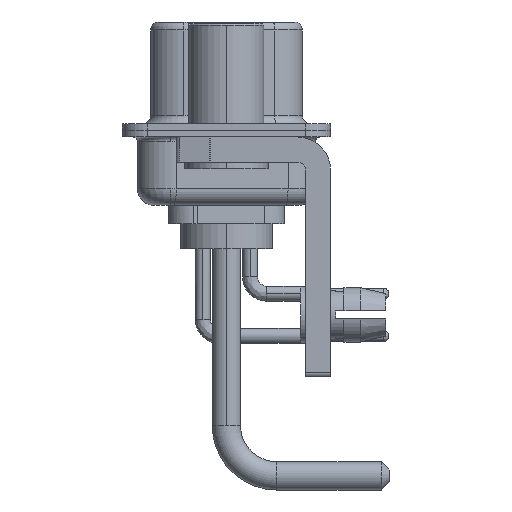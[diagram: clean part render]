
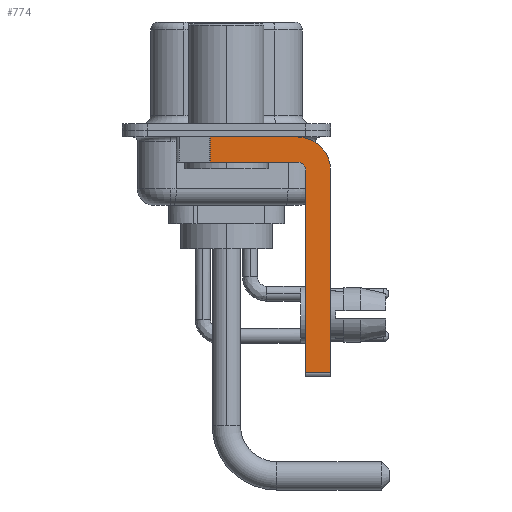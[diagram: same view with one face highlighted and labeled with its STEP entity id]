
A CAD part, left-side view. The second image highlights one B-rep face of the part: STEP entity #774.
In plain terms, the highlighted planar face has unit normal (-1, 0, 0).
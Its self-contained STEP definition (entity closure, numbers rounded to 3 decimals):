
#564 = DIRECTION ( 'NONE',  ( 0., 0., 1. ) ) ;
#774 = ADVANCED_FACE ( 'NONE', ( #10113 ), #27940, .F. ) ;
#1044 = LINE ( 'NONE', #5368, #12003 ) ;
#1234 = ORIENTED_EDGE ( 'NONE', *, *, #3634, .F. ) ;
#1463 = CARTESIAN_POINT ( 'NONE',  ( -2.9, -4.25, -2.4 ) ) ;
#1567 = VERTEX_POINT ( 'NONE', #2811 ) ;
#2404 = AXIS2_PLACEMENT_3D ( 'NONE', #1463, #26087, #26253 ) ;
#2811 = CARTESIAN_POINT ( 'NONE',  ( -2.9, -4.25, -0.4 ) ) ;
#2847 = DIRECTION ( 'NONE',  ( 0., 0., -1. ) ) ;
#3634 = EDGE_CURVE ( 'NONE', #18021, #13394, #13220, .T. ) ;
#4487 = CARTESIAN_POINT ( 'NONE',  ( -2.9, -4.25, -2.4 ) ) ;
#4688 = CARTESIAN_POINT ( 'NONE',  ( -2.9, -4.25, -2.4 ) ) ;
#5109 = CARTESIAN_POINT ( 'NONE',  ( -2.9, -4.25, -1.9 ) ) ;
#5368 = CARTESIAN_POINT ( 'NONE',  ( -2.9, -4.75, -14.8 ) ) ;
#6157 = CARTESIAN_POINT ( 'NONE',  ( -2.9, -4.25, -1.9 ) ) ;
#6579 = ORIENTED_EDGE ( 'NONE', *, *, #14877, .F. ) ;
#6624 = DIRECTION ( 'NONE',  ( 0., -1., 0. ) ) ;
#7213 = ORIENTED_EDGE ( 'NONE', *, *, #32289, .F. ) ;
#7903 = VERTEX_POINT ( 'NONE', #11175 ) ;
#8265 = DIRECTION ( 'NONE',  ( 0., 0., -1. ) ) ;
#8285 = AXIS2_PLACEMENT_3D ( 'NONE', #4688, #25480, #2847 ) ;
#8656 = ORIENTED_EDGE ( 'NONE', *, *, #25302, .T. ) ;
#8937 = LINE ( 'NONE', #11593, #17824 ) ;
#9923 = EDGE_CURVE ( 'NONE', #20042, #30696, #11492, .T. ) ;
#10113 = FACE_OUTER_BOUND ( 'NONE', #10461, .T. ) ;
#10461 = EDGE_LOOP ( 'NONE', ( #28764, #23214, #7213, #27633, #17973, #8656, #1234, #6579 ) ) ;
#10996 = VECTOR ( 'NONE', #23599, 1000. ) ;
#11175 = CARTESIAN_POINT ( 'NONE',  ( -2.9, -4.75, -14.55 ) ) ;
#11492 = LINE ( 'NONE', #26179, #30170 ) ;
#11593 = CARTESIAN_POINT ( 'NONE',  ( -2.9, 3., -0.4 ) ) ;
#12003 = VECTOR ( 'NONE', #564, 1000. ) ;
#13220 = LINE ( 'NONE', #27942, #19456 ) ;
#13394 = VERTEX_POINT ( 'NONE', #15783 ) ;
#14877 = EDGE_CURVE ( 'NONE', #1567, #18021, #15669, .T. ) ;
#15023 = LINE ( 'NONE', #5109, #27027 ) ;
#15160 = EDGE_CURVE ( 'NONE', #29015, #21224, #16746, .T. ) ;
#15669 = CIRCLE ( 'NONE', #8285, 2. ) ;
#15738 = CARTESIAN_POINT ( 'NONE',  ( -2.9, 0.978, -0.4 ) ) ;
#15783 = CARTESIAN_POINT ( 'NONE',  ( -2.9, -6.25, -14.55 ) ) ;
#16746 = CIRCLE ( 'NONE', #17805, 0.5 ) ;
#16793 = EDGE_CURVE ( 'NONE', #7903, #29015, #1044, .T. ) ;
#17805 = AXIS2_PLACEMENT_3D ( 'NONE', #4487, #26945, #26785 ) ;
#17824 = VECTOR ( 'NONE', #6624, 1000. ) ;
#17973 = ORIENTED_EDGE ( 'NONE', *, *, #16793, .F. ) ;
#18021 = VERTEX_POINT ( 'NONE', #31630 ) ;
#18334 = LINE ( 'NONE', #28401, #10996 ) ;
#19456 = VECTOR ( 'NONE', #8265, 1000. ) ;
#20042 = VERTEX_POINT ( 'NONE', #15738 ) ;
#21224 = VERTEX_POINT ( 'NONE', #6157 ) ;
#23214 = ORIENTED_EDGE ( 'NONE', *, *, #9923, .T. ) ;
#23441 = CARTESIAN_POINT ( 'NONE',  ( -2.9, 0.978, -1.9 ) ) ;
#23599 = DIRECTION ( 'NONE',  ( 0., -1., 0. ) ) ;
#23841 = CARTESIAN_POINT ( 'NONE',  ( -2.9, -4.75, -2.4 ) ) ;
#24779 = EDGE_CURVE ( 'NONE', #20042, #1567, #8937, .T. ) ;
#25302 = EDGE_CURVE ( 'NONE', #7903, #13394, #18334, .T. ) ;
#25480 = DIRECTION ( 'NONE',  ( 1., 0., 0. ) ) ;
#26087 = DIRECTION ( 'NONE',  ( 1., 0., 0. ) ) ;
#26179 = CARTESIAN_POINT ( 'NONE',  ( -2.9, 0.978, -1.9 ) ) ;
#26253 = DIRECTION ( 'NONE',  ( 0., 0., -1. ) ) ;
#26785 = DIRECTION ( 'NONE',  ( 0., 0., 1. ) ) ;
#26945 = DIRECTION ( 'NONE',  ( -1., 0., 0. ) ) ;
#27027 = VECTOR ( 'NONE', #27573, 1000. ) ;
#27573 = DIRECTION ( 'NONE',  ( 0., 1., 0. ) ) ;
#27633 = ORIENTED_EDGE ( 'NONE', *, *, #15160, .F. ) ;
#27940 = PLANE ( 'NONE',  #2404 ) ;
#27942 = CARTESIAN_POINT ( 'NONE',  ( -2.9, -6.25, -2.4 ) ) ;
#28401 = CARTESIAN_POINT ( 'NONE',  ( -2.9, -4.25, -14.55 ) ) ;
#28764 = ORIENTED_EDGE ( 'NONE', *, *, #24779, .F. ) ;
#29015 = VERTEX_POINT ( 'NONE', #23841 ) ;
#30170 = VECTOR ( 'NONE', #31140, 1000. ) ;
#30696 = VERTEX_POINT ( 'NONE', #23441 ) ;
#31140 = DIRECTION ( 'NONE',  ( 0., 0., -1. ) ) ;
#31630 = CARTESIAN_POINT ( 'NONE',  ( -2.9, -6.25, -2.4 ) ) ;
#32289 = EDGE_CURVE ( 'NONE', #21224, #30696, #15023, .T. ) ;
